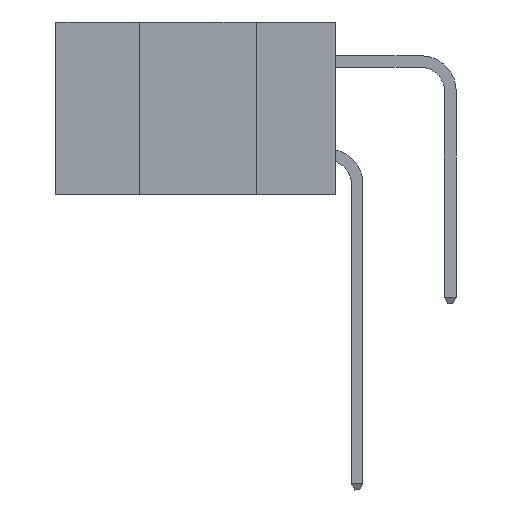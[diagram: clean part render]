
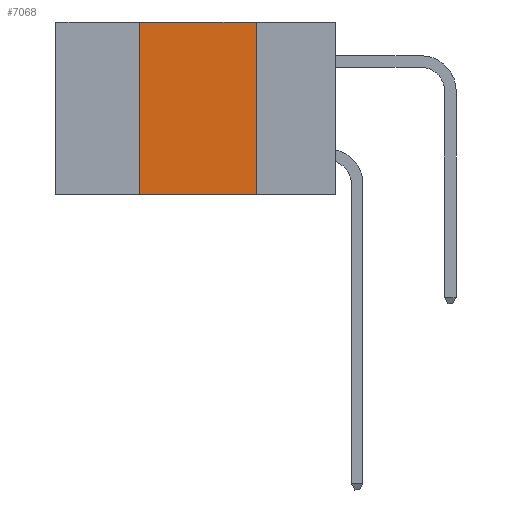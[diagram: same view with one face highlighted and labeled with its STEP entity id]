
A CAD part, left-side view. The second image highlights one B-rep face of the part: STEP entity #7068.
In plain terms, the highlighted planar face has unit normal (-1, 0, 0).
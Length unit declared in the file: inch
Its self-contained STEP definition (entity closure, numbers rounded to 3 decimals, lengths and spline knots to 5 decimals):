
#7 = VECTOR ( 'NONE', #18088, 39.37008 ) ;
#713 = CARTESIAN_POINT ( 'NONE',  ( 0., 0.17, -0.37 ) ) ;
#1755 = DIRECTION ( 'NONE',  ( 0., 0., 1. ) ) ;
#2728 = CARTESIAN_POINT ( 'NONE',  ( 0., 0.42, -0.37 ) ) ;
#2790 = CARTESIAN_POINT ( 'NONE',  ( 0., 0.42, 0. ) ) ;
#3554 = EDGE_CURVE ( 'NONE', #25435, #11509, #29203, .T. ) ;
#3568 = ORIENTED_EDGE ( 'NONE', *, *, #9155, .T. ) ;
#3702 = LINE ( 'NONE', #20659, #19816 ) ;
#3908 = VERTEX_POINT ( 'NONE', #2790 ) ;
#3910 = CARTESIAN_POINT ( 'NONE',  ( 0., 0.6, 0. ) ) ;
#6214 = ORIENTED_EDGE ( 'NONE', *, *, #17939, .F. ) ;
#6789 = FACE_OUTER_BOUND ( 'NONE', #11010, .T. ) ;
#7068 = ADVANCED_FACE ( 'NONE', ( #6789 ), #17039, .F. ) ;
#7383 = EDGE_CURVE ( 'NONE', #3908, #25435, #8542, .T. ) ;
#7653 = DIRECTION ( 'NONE',  ( 0., 0., -1. ) ) ;
#8542 = LINE ( 'NONE', #3910, #9313 ) ;
#9155 = EDGE_CURVE ( 'NONE', #15263, #11509, #9526, .T. ) ;
#9313 = VECTOR ( 'NONE', #29945, 39.37008 ) ;
#9526 = LINE ( 'NONE', #27223, #7 ) ;
#11010 = EDGE_LOOP ( 'NONE', ( #20336, #21022, #6214, #3568 ) ) ;
#11509 = VERTEX_POINT ( 'NONE', #713 ) ;
#13031 = DIRECTION ( 'NONE',  ( 0., 0., -1. ) ) ;
#15263 = VERTEX_POINT ( 'NONE', #2728 ) ;
#17039 = PLANE ( 'NONE',  #29406 ) ;
#17939 = EDGE_CURVE ( 'NONE', #15263, #3908, #3702, .T. ) ;
#18088 = DIRECTION ( 'NONE',  ( 0., -1., 0. ) ) ;
#18740 = CARTESIAN_POINT ( 'NONE',  ( 0., 0.17, 0. ) ) ;
#19816 = VECTOR ( 'NONE', #1755, 39.37008 ) ;
#20046 = VECTOR ( 'NONE', #7653, 39.37008 ) ;
#20336 = ORIENTED_EDGE ( 'NONE', *, *, #3554, .F. ) ;
#20659 = CARTESIAN_POINT ( 'NONE',  ( 0., 0.42, 0. ) ) ;
#21022 = ORIENTED_EDGE ( 'NONE', *, *, #7383, .F. ) ;
#24531 = CARTESIAN_POINT ( 'NONE',  ( 0., 0.6, 0. ) ) ;
#25435 = VERTEX_POINT ( 'NONE', #18740 ) ;
#26865 = DIRECTION ( 'NONE',  ( 1., 0., 0. ) ) ;
#27223 = CARTESIAN_POINT ( 'NONE',  ( 0., 0.6, -0.37 ) ) ;
#27632 = CARTESIAN_POINT ( 'NONE',  ( 0., 0.17, 0. ) ) ;
#29203 = LINE ( 'NONE', #27632, #20046 ) ;
#29406 = AXIS2_PLACEMENT_3D ( 'NONE', #24531, #26865, #13031 ) ;
#29945 = DIRECTION ( 'NONE',  ( 0., -1., 0. ) ) ;
